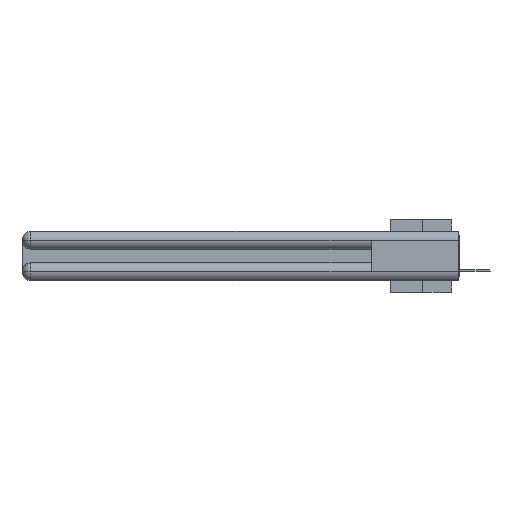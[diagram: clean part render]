
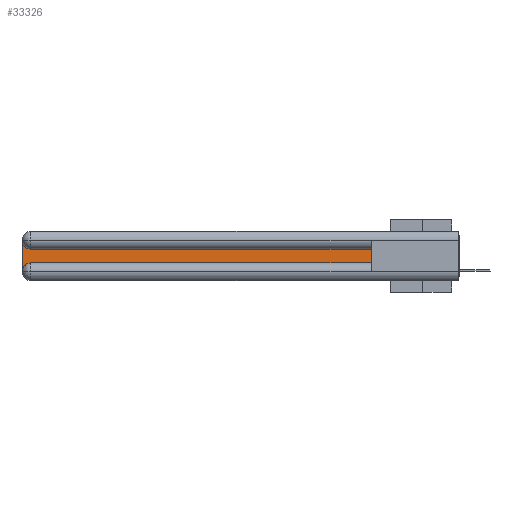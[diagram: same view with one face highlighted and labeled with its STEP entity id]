
A CAD part, left-side view. The second image highlights one B-rep face of the part: STEP entity #33326.
In plain terms, the highlighted planar face has unit normal (-1, 0, 0).
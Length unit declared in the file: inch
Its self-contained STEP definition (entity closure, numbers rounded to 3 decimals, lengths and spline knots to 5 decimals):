
#19 = CARTESIAN_POINT ( 'NONE',  ( 0.075, 3., -0.2775 ) ) ;
#1702 = LINE ( 'NONE', #7087, #29500 ) ;
#1914 = EDGE_CURVE ( 'NONE', #15432, #23110, #2900, .T. ) ;
#2162 = EDGE_LOOP ( 'NONE', ( #8856, #27469, #16610, #17290, #22466, #4919 ) ) ;
#2178 = VECTOR ( 'NONE', #22947, 39.37008 ) ;
#2615 = CARTESIAN_POINT ( 'NONE',  ( 0.075, 3., -0.2175 ) ) ;
#2821 = DIRECTION ( 'NONE',  ( 0., 0., -1. ) ) ;
#2900 = LINE ( 'NONE', #17504, #20686 ) ;
#3160 = DIRECTION ( 'NONE',  ( 0., 0., -1. ) ) ;
#3332 = CARTESIAN_POINT ( 'NONE',  ( 0.075, 3., -0.0625 ) ) ;
#4008 = VERTEX_POINT ( 'NONE', #19 ) ;
#4919 = ORIENTED_EDGE ( 'NONE', *, *, #24559, .T. ) ;
#6799 = AXIS2_PLACEMENT_3D ( 'NONE', #10655, #13483, #3160 ) ;
#6902 = CIRCLE ( 'NONE', #32016, 0.06 ) ;
#7087 = CARTESIAN_POINT ( 'NONE',  ( 0.075, 0.6, -0.2175 ) ) ;
#7663 = CARTESIAN_POINT ( 'NONE',  ( 0.075, 0.6, -0.2175 ) ) ;
#8856 = ORIENTED_EDGE ( 'NONE', *, *, #1914, .T. ) ;
#9640 = VERTEX_POINT ( 'NONE', #3332 ) ;
#9692 = DIRECTION ( 'NONE',  ( 0., 0., -1. ) ) ;
#10655 = CARTESIAN_POINT ( 'NONE',  ( 0.075, 3., -0.1225 ) ) ;
#11002 = CARTESIAN_POINT ( 'NONE',  ( 0.075, 2.94, -0.1225 ) ) ;
#11890 = LINE ( 'NONE', #7663, #2178 ) ;
#12084 = DIRECTION ( 'NONE',  ( 1., 0., 0. ) ) ;
#12114 = EDGE_CURVE ( 'NONE', #23110, #9640, #6902, .T. ) ;
#13321 = AXIS2_PLACEMENT_3D ( 'NONE', #32564, #12084, #22187 ) ;
#13483 = DIRECTION ( 'NONE',  ( 1., 0., 0. ) ) ;
#13664 = VECTOR ( 'NONE', #2821, 39.37008 ) ;
#14823 = CARTESIAN_POINT ( 'NONE',  ( 0.075, 2.94, -0.2175 ) ) ;
#15432 = VERTEX_POINT ( 'NONE', #31634 ) ;
#15595 = EDGE_CURVE ( 'NONE', #4008, #27495, #20714, .T. ) ;
#15894 = CARTESIAN_POINT ( 'NONE',  ( 0.075, 2.94, -0.0625 ) ) ;
#16610 = ORIENTED_EDGE ( 'NONE', *, *, #17240, .T. ) ;
#17240 = EDGE_CURVE ( 'NONE', #9640, #4008, #31365, .T. ) ;
#17290 = ORIENTED_EDGE ( 'NONE', *, *, #15595, .T. ) ;
#17504 = CARTESIAN_POINT ( 'NONE',  ( 0.075, 0.6, -0.1225 ) ) ;
#20686 = VECTOR ( 'NONE', #25459, 39.37008 ) ;
#20714 = CIRCLE ( 'NONE', #13321, 0.06 ) ;
#22187 = DIRECTION ( 'NONE',  ( 0., 0., -1. ) ) ;
#22466 = ORIENTED_EDGE ( 'NONE', *, *, #26299, .T. ) ;
#22947 = DIRECTION ( 'NONE',  ( 0., 0., 1. ) ) ;
#23110 = VERTEX_POINT ( 'NONE', #11002 ) ;
#24559 = EDGE_CURVE ( 'NONE', #26423, #15432, #11890, .T. ) ;
#24990 = DIRECTION ( 'NONE',  ( 0., -1., 0. ) ) ;
#25459 = DIRECTION ( 'NONE',  ( 0., 1., 0. ) ) ;
#26299 = EDGE_CURVE ( 'NONE', #27495, #26423, #1702, .T. ) ;
#26423 = VERTEX_POINT ( 'NONE', #33116 ) ;
#27469 = ORIENTED_EDGE ( 'NONE', *, *, #12114, .T. ) ;
#27495 = VERTEX_POINT ( 'NONE', #14823 ) ;
#29003 = PLANE ( 'NONE',  #6799 ) ;
#29500 = VECTOR ( 'NONE', #24990, 39.37008 ) ;
#31365 = LINE ( 'NONE', #2615, #13664 ) ;
#31634 = CARTESIAN_POINT ( 'NONE',  ( 0.075, 0.6, -0.1225 ) ) ;
#31851 = DIRECTION ( 'NONE',  ( 1., 0., 0. ) ) ;
#32016 = AXIS2_PLACEMENT_3D ( 'NONE', #15894, #31851, #9692 ) ;
#32564 = CARTESIAN_POINT ( 'NONE',  ( 0.075, 2.94, -0.2775 ) ) ;
#32767 = FACE_OUTER_BOUND ( 'NONE', #2162, .T. ) ;
#33116 = CARTESIAN_POINT ( 'NONE',  ( 0.075, 0.6, -0.2175 ) ) ;
#33326 = ADVANCED_FACE ( 'NONE', ( #32767 ), #29003, .F. ) ;
